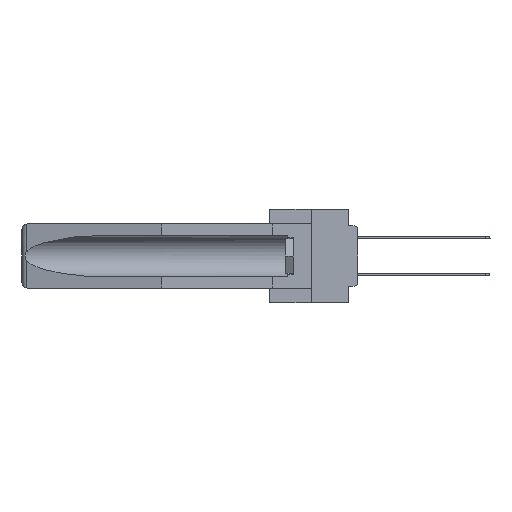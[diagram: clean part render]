
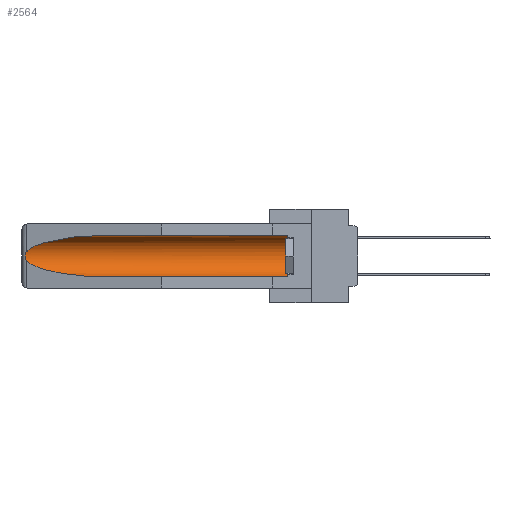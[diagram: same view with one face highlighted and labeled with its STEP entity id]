
A CAD part, left-side view. The second image highlights one B-rep face of the part: STEP entity #2564.
In plain terms, the highlighted cylindrical face has radius 2.857 mm (diameter 5.715 mm), a partial arc.
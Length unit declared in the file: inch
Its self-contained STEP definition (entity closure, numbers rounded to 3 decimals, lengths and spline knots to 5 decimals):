
#124 = VERTEX_POINT ( 'NONE', #30244 ) ;
#354 = EDGE_CURVE ( 'NONE', #18548, #27156, #14026, .T. ) ;
#633 = CARTESIAN_POINT ( 'NONE',  ( 0.2675, 1.53308, -0.17534 ) ) ;
#1470 = DIRECTION ( 'NONE',  ( 0., -1., 0. ) ) ;
#1971 = ORIENTED_EDGE ( 'NONE', *, *, #28961, .T. ) ;
#1998 = CARTESIAN_POINT ( 'NONE',  ( 0.21114, 1.30732, -0.059 ) ) ;
#2564 = ADVANCED_FACE ( 'NONE', ( #7312 ), #16809, .F. ) ;
#3204 = CARTESIAN_POINT ( 'NONE',  ( 0.155, 1.07973, -0.284 ) ) ;
#3895 = CARTESIAN_POINT ( 'NONE',  ( 0.26537, 1.52718, -0.14972 ) ) ;
#4897 = B_SPLINE_CURVE_WITH_KNOTS ( 'NONE', 3,
 ( #27615, #17611, #10801, #20468, #7787, #633, #17454, #30156, #5417, #8414 ),
 .UNSPECIFIED., .F., .F.,
 ( 4, 2, 2, 2, 4 ),
 ( 0., 0.00029, 0.00058, 0.00087, 0.00117 ),
 .UNSPECIFIED. ) ;
#5129 =( BOUNDED_CURVE ( )  B_SPLINE_CURVE ( 3, ( #12679, #29496, #27101, #7766 ),
 .UNSPECIFIED., .F., .F. ) 
 B_SPLINE_CURVE_WITH_KNOTS ( ( 4, 4 ),
 ( 0.1948, 1.5708 ),
 .UNSPECIFIED. ) 
 CURVE ( )  GEOMETRIC_REPRESENTATION_ITEM ( )  RATIONAL_B_SPLINE_CURVE ( ( 1., 0.848, 0.848, 1. ) ) 
 REPRESENTATION_ITEM ( '' )  );
#5417 = CARTESIAN_POINT ( 'NONE',  ( 0.26597, 1.5296, -0.19026 ) ) ;
#5618 = CIRCLE ( 'NONE', #28932, 0.1125 ) ;
#5733 = LINE ( 'NONE', #15692, #23796 ) ;
#6187 = EDGE_CURVE ( 'NONE', #30782, #27910, #5129, .T. ) ;
#7312 = FACE_OUTER_BOUND ( 'NONE', #7714, .T. ) ;
#7714 = EDGE_LOOP ( 'NONE', ( #11128, #30491, #16503, #30343, #21280, #1971 ) ) ;
#7766 = CARTESIAN_POINT ( 'NONE',  ( 0.155, 1.07973, -0.284 ) ) ;
#7787 = CARTESIAN_POINT ( 'NONE',  ( 0.2675, 1.53308, -0.16763 ) ) ;
#8414 = CARTESIAN_POINT ( 'NONE',  ( 0.26537, 1.52718, -0.19328 ) ) ;
#8823 = EDGE_CURVE ( 'NONE', #124, #27910, #30649, .T. ) ;
#9221 = EDGE_CURVE ( 'NONE', #27156, #30782, #4897, .T. ) ;
#9385 = DIRECTION ( 'NONE',  ( 0., 1., 0. ) ) ;
#10443 = CARTESIAN_POINT ( 'NONE',  ( 0.155, 1.07973, -0.059 ) ) ;
#10801 = CARTESIAN_POINT ( 'NONE',  ( 0.26654, 1.53092, -0.15636 ) ) ;
#11128 = ORIENTED_EDGE ( 'NONE', *, *, #354, .T. ) ;
#11857 = VECTOR ( 'NONE', #9385, 39.37008 ) ;
#12679 = CARTESIAN_POINT ( 'NONE',  ( 0.26537, 1.52718, -0.19328 ) ) ;
#12822 = AXIS2_PLACEMENT_3D ( 'NONE', #24265, #26960, #24423 ) ;
#13159 = CARTESIAN_POINT ( 'NONE',  ( 0.26537, 1.52718, -0.14972 ) ) ;
#14026 =( BOUNDED_CURVE ( )  B_SPLINE_CURVE ( 3, ( #23708, #1998, #30553, #3895 ),
 .UNSPECIFIED., .F., .F. ) 
 B_SPLINE_CURVE_WITH_KNOTS ( ( 4, 4 ),
 ( 4.71239, 6.08839 ),
 .UNSPECIFIED. ) 
 CURVE ( )  GEOMETRIC_REPRESENTATION_ITEM ( )  RATIONAL_B_SPLINE_CURVE ( ( 1., 0.848, 0.848, 1. ) ) 
 REPRESENTATION_ITEM ( '' )  );
#15692 = CARTESIAN_POINT ( 'NONE',  ( 0.155, -0.30754, -0.059 ) ) ;
#15891 = CARTESIAN_POINT ( 'NONE',  ( 0.155, 0.126, -0.1715 ) ) ;
#16503 = ORIENTED_EDGE ( 'NONE', *, *, #6187, .T. ) ;
#16809 = CYLINDRICAL_SURFACE ( 'NONE', #12822, 0.1125 ) ;
#17454 = CARTESIAN_POINT ( 'NONE',  ( 0.2673, 1.53269, -0.17917 ) ) ;
#17611 = CARTESIAN_POINT ( 'NONE',  ( 0.26597, 1.52961, -0.15275 ) ) ;
#18548 = VERTEX_POINT ( 'NONE', #10443 ) ;
#18572 = DIRECTION ( 'NONE',  ( 0., 0., 1. ) ) ;
#19783 = CARTESIAN_POINT ( 'NONE',  ( 0.26537, 1.52718, -0.19328 ) ) ;
#19981 = DIRECTION ( 'NONE',  ( 0., 1., 0. ) ) ;
#20016 = CARTESIAN_POINT ( 'NONE',  ( 0.155, 0.126, -0.059 ) ) ;
#20468 = CARTESIAN_POINT ( 'NONE',  ( 0.2673, 1.5327, -0.16383 ) ) ;
#21280 = ORIENTED_EDGE ( 'NONE', *, *, #30000, .T. ) ;
#23708 = CARTESIAN_POINT ( 'NONE',  ( 0.155, 1.07973, -0.059 ) ) ;
#23796 = VECTOR ( 'NONE', #19981, 39.37008 ) ;
#24265 = CARTESIAN_POINT ( 'NONE',  ( 0.155, -0.30754, -0.1715 ) ) ;
#24423 = DIRECTION ( 'NONE',  ( 0., 0., 1. ) ) ;
#26198 = CARTESIAN_POINT ( 'NONE',  ( 0.155, -0.30754, -0.284 ) ) ;
#26960 = DIRECTION ( 'NONE',  ( 0., 1., 0. ) ) ;
#27101 = CARTESIAN_POINT ( 'NONE',  ( 0.21114, 1.30732, -0.284 ) ) ;
#27156 = VERTEX_POINT ( 'NONE', #13159 ) ;
#27615 = CARTESIAN_POINT ( 'NONE',  ( 0.26537, 1.52718, -0.14972 ) ) ;
#27910 = VERTEX_POINT ( 'NONE', #3204 ) ;
#28587 = VERTEX_POINT ( 'NONE', #20016 ) ;
#28932 = AXIS2_PLACEMENT_3D ( 'NONE', #15891, #1470, #18572 ) ;
#28961 = EDGE_CURVE ( 'NONE', #28587, #18548, #5733, .T. ) ;
#29496 = CARTESIAN_POINT ( 'NONE',  ( 0.25451, 1.48313, -0.24835 ) ) ;
#30000 = EDGE_CURVE ( 'NONE', #124, #28587, #5618, .T. ) ;
#30156 = CARTESIAN_POINT ( 'NONE',  ( 0.26655, 1.53094, -0.18657 ) ) ;
#30244 = CARTESIAN_POINT ( 'NONE',  ( 0.155, 0.126, -0.284 ) ) ;
#30343 = ORIENTED_EDGE ( 'NONE', *, *, #8823, .F. ) ;
#30491 = ORIENTED_EDGE ( 'NONE', *, *, #9221, .T. ) ;
#30553 = CARTESIAN_POINT ( 'NONE',  ( 0.25451, 1.48313, -0.09465 ) ) ;
#30649 = LINE ( 'NONE', #26198, #11857 ) ;
#30782 = VERTEX_POINT ( 'NONE', #19783 ) ;
